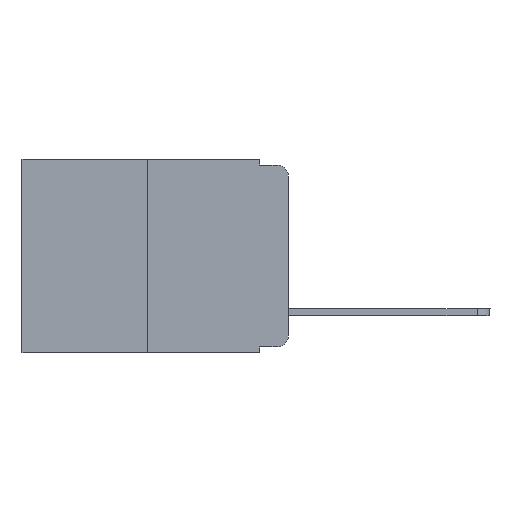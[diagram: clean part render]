
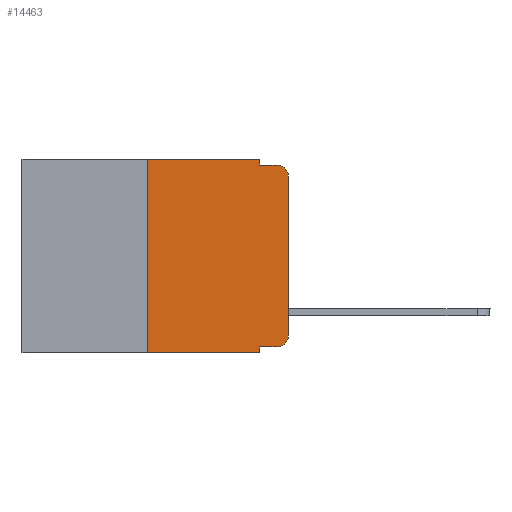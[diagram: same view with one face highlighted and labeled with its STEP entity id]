
A CAD part, left-side view. The second image highlights one B-rep face of the part: STEP entity #14463.
In plain terms, the highlighted planar face has unit normal (-1, 0, 0).
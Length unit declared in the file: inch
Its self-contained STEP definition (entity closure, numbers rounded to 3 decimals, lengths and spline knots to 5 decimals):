
#60 = CARTESIAN_POINT ( 'NONE',  ( 0., 0.473, 0. ) ) ;
#524 = CARTESIAN_POINT ( 'NONE',  ( 0., 0.473, 0. ) ) ;
#610 = VERTEX_POINT ( 'NONE', #19864 ) ;
#642 = DIRECTION ( 'NONE',  ( 1., 0., 0. ) ) ;
#721 = CARTESIAN_POINT ( 'NONE',  ( 0., 0.051, -0.333 ) ) ;
#1005 = VERTEX_POINT ( 'NONE', #15404 ) ;
#1068 = EDGE_CURVE ( 'NONE', #1005, #19128, #8716, .T. ) ;
#1447 = DIRECTION ( 'NONE',  ( 0., 0., -1. ) ) ;
#1576 = VECTOR ( 'NONE', #21596, 39.37008 ) ;
#1644 = VERTEX_POINT ( 'NONE', #15818 ) ;
#1675 = DIRECTION ( 'NONE',  ( 0., -1., 0. ) ) ;
#2053 = CARTESIAN_POINT ( 'NONE',  ( 0., 0.25, 0. ) ) ;
#2167 = ORIENTED_EDGE ( 'NONE', *, *, #7673, .T. ) ;
#2239 = FACE_OUTER_BOUND ( 'NONE', #10791, .T. ) ;
#2299 = VECTOR ( 'NONE', #14301, 39.37008 ) ;
#2526 = CARTESIAN_POINT ( 'NONE',  ( 0., 0., 0. ) ) ;
#3578 = VERTEX_POINT ( 'NONE', #12034 ) ;
#3585 = ORIENTED_EDGE ( 'NONE', *, *, #18171, .F. ) ;
#3636 = DIRECTION ( 'NONE',  ( 0., 0., 1. ) ) ;
#3692 = LINE ( 'NONE', #9570, #1576 ) ;
#4323 = CARTESIAN_POINT ( 'NONE',  ( 0., 0.02, -0.333 ) ) ;
#4709 = VERTEX_POINT ( 'NONE', #4323 ) ;
#5230 = ORIENTED_EDGE ( 'NONE', *, *, #12856, .F. ) ;
#5400 = EDGE_CURVE ( 'NONE', #20713, #4709, #19900, .T. ) ;
#6110 = ORIENTED_EDGE ( 'NONE', *, *, #13463, .T. ) ;
#6553 = CARTESIAN_POINT ( 'NONE',  ( 0., 0.02, -0.01 ) ) ;
#6573 = CARTESIAN_POINT ( 'NONE',  ( 0., 0.02, -0.313 ) ) ;
#6872 = CARTESIAN_POINT ( 'NONE',  ( 0., 0.473, -0.343 ) ) ;
#7338 = AXIS2_PLACEMENT_3D ( 'NONE', #524, #642, #21413 ) ;
#7655 = DIRECTION ( 'NONE',  ( 0., -1., 0. ) ) ;
#7673 = EDGE_CURVE ( 'NONE', #4709, #16037, #11117, .T. ) ;
#8155 = CARTESIAN_POINT ( 'NONE',  ( 0., 0.051, -0.333 ) ) ;
#8365 = EDGE_CURVE ( 'NONE', #16037, #1644, #11275, .T. ) ;
#8584 = AXIS2_PLACEMENT_3D ( 'NONE', #6573, #20423, #9884 ) ;
#8716 = LINE ( 'NONE', #10523, #19511 ) ;
#8868 = LINE ( 'NONE', #15892, #2299 ) ;
#9570 = CARTESIAN_POINT ( 'NONE',  ( 0., 0.051, 0. ) ) ;
#9599 = VECTOR ( 'NONE', #7655, 39.37008 ) ;
#9884 = DIRECTION ( 'NONE',  ( 0., 0., -1. ) ) ;
#10236 = CIRCLE ( 'NONE', #16016, 0.02 ) ;
#10484 = ORIENTED_EDGE ( 'NONE', *, *, #15731, .F. ) ;
#10523 = CARTESIAN_POINT ( 'NONE',  ( 0., 0.051, 0. ) ) ;
#10586 = VECTOR ( 'NONE', #3636, 39.37008 ) ;
#10791 = EDGE_LOOP ( 'NONE', ( #13037, #12765, #10484, #18824, #3585, #5230, #6110, #11665, #14458, #2167 ) ) ;
#11117 = CIRCLE ( 'NONE', #8584, 0.02 ) ;
#11275 = LINE ( 'NONE', #2526, #16549 ) ;
#11665 = ORIENTED_EDGE ( 'NONE', *, *, #18333, .F. ) ;
#11888 = DIRECTION ( 'NONE',  ( 0., -1., 0. ) ) ;
#12034 = CARTESIAN_POINT ( 'NONE',  ( 0., 0.25, -0.343 ) ) ;
#12765 = ORIENTED_EDGE ( 'NONE', *, *, #12934, .T. ) ;
#12856 = EDGE_CURVE ( 'NONE', #3578, #17039, #17492, .T. ) ;
#12934 = EDGE_CURVE ( 'NONE', #1644, #19289, #10236, .T. ) ;
#13037 = ORIENTED_EDGE ( 'NONE', *, *, #8365, .T. ) ;
#13353 = LINE ( 'NONE', #6872, #14179 ) ;
#13463 = EDGE_CURVE ( 'NONE', #3578, #610, #13353, .T. ) ;
#13698 = LINE ( 'NONE', #60, #17497 ) ;
#14179 = VECTOR ( 'NONE', #11888, 39.37008 ) ;
#14301 = DIRECTION ( 'NONE',  ( 0., -1., 0. ) ) ;
#14458 = ORIENTED_EDGE ( 'NONE', *, *, #5400, .T. ) ;
#14463 = ADVANCED_FACE ( 'NONE', ( #2239 ), #18022, .F. ) ;
#14862 = CARTESIAN_POINT ( 'NONE',  ( 0., 0.02, -0.03 ) ) ;
#15404 = CARTESIAN_POINT ( 'NONE',  ( 0., 0.051, 0. ) ) ;
#15731 = EDGE_CURVE ( 'NONE', #19128, #19289, #8868, .T. ) ;
#15818 = CARTESIAN_POINT ( 'NONE',  ( 0., 0., -0.03 ) ) ;
#15892 = CARTESIAN_POINT ( 'NONE',  ( 0., 0.051, -0.01 ) ) ;
#16016 = AXIS2_PLACEMENT_3D ( 'NONE', #14862, #18158, #19743 ) ;
#16037 = VERTEX_POINT ( 'NONE', #22352 ) ;
#16549 = VECTOR ( 'NONE', #17979, 39.37008 ) ;
#17039 = VERTEX_POINT ( 'NONE', #2053 ) ;
#17143 = CARTESIAN_POINT ( 'NONE',  ( 0., 0.051, -0.01 ) ) ;
#17492 = LINE ( 'NONE', #21118, #10586 ) ;
#17497 = VECTOR ( 'NONE', #1675, 39.37008 ) ;
#17979 = DIRECTION ( 'NONE',  ( 0., 0., 1. ) ) ;
#18022 = PLANE ( 'NONE',  #7338 ) ;
#18158 = DIRECTION ( 'NONE',  ( -1., 0., 0. ) ) ;
#18171 = EDGE_CURVE ( 'NONE', #17039, #1005, #13698, .T. ) ;
#18333 = EDGE_CURVE ( 'NONE', #20713, #610, #3692, .T. ) ;
#18824 = ORIENTED_EDGE ( 'NONE', *, *, #1068, .F. ) ;
#19128 = VERTEX_POINT ( 'NONE', #17143 ) ;
#19289 = VERTEX_POINT ( 'NONE', #6553 ) ;
#19511 = VECTOR ( 'NONE', #1447, 39.37008 ) ;
#19743 = DIRECTION ( 'NONE',  ( 0., 0., -1. ) ) ;
#19864 = CARTESIAN_POINT ( 'NONE',  ( 0., 0.051, -0.343 ) ) ;
#19900 = LINE ( 'NONE', #721, #9599 ) ;
#20423 = DIRECTION ( 'NONE',  ( -1., 0., 0. ) ) ;
#20713 = VERTEX_POINT ( 'NONE', #8155 ) ;
#21118 = CARTESIAN_POINT ( 'NONE',  ( 0., 0.25, 0. ) ) ;
#21413 = DIRECTION ( 'NONE',  ( 0., 0., -1. ) ) ;
#21596 = DIRECTION ( 'NONE',  ( 0., 0., -1. ) ) ;
#22352 = CARTESIAN_POINT ( 'NONE',  ( 0., 0., -0.313 ) ) ;
